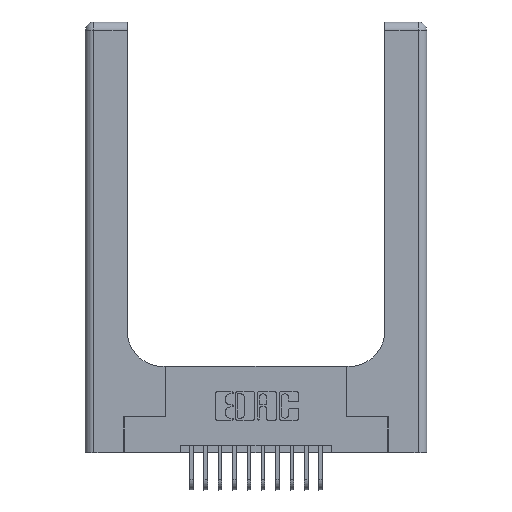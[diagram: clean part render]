
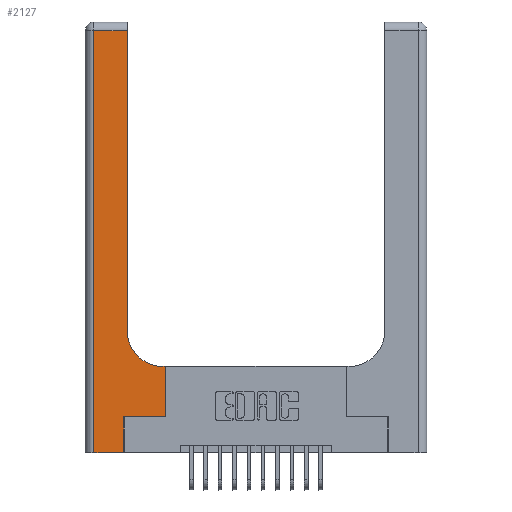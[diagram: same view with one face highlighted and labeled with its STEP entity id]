
A CAD part, top view. The second image highlights one B-rep face of the part: STEP entity #2127.
In plain terms, the highlighted planar face has unit normal (0, 0, 1).
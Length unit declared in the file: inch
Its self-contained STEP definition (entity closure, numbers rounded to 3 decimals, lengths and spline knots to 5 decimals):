
#463 = VERTEX_POINT ( 'NONE', #16548 ) ;
#672 = VERTEX_POINT ( 'NONE', #14677 ) ;
#1112 = VERTEX_POINT ( 'NONE', #16464 ) ;
#1236 = VECTOR ( 'NONE', #17780, 39.37008 ) ;
#1270 = CARTESIAN_POINT ( 'NONE',  ( 0.269, 0., 0.37 ) ) ;
#1528 = EDGE_CURVE ( 'NONE', #463, #9637, #14666, .T. ) ;
#1579 = VECTOR ( 'NONE', #14636, 39.37008 ) ;
#1701 = VECTOR ( 'NONE', #14413, 39.37008 ) ;
#1878 = VERTEX_POINT ( 'NONE', #7580 ) ;
#2127 = ADVANCED_FACE ( 'NONE', ( #17634 ), #6826, .F. ) ;
#2381 = LINE ( 'NONE', #10293, #9629 ) ;
#2548 = EDGE_CURVE ( 'NONE', #1112, #5466, #13866, .T. ) ;
#2613 = EDGE_LOOP ( 'NONE', ( #13103, #8641, #13406, #6641, #18690, #15716, #16175, #10915, #14862 ) ) ;
#3111 = VECTOR ( 'NONE', #7740, 39.37008 ) ;
#3195 = DIRECTION ( 'NONE',  ( -1., 0., 0. ) ) ;
#3203 = VECTOR ( 'NONE', #11678, 39.37008 ) ;
#3715 = VERTEX_POINT ( 'NONE', #17293 ) ;
#4484 = CARTESIAN_POINT ( 'NONE',  ( 0.5585, 0.25, 0.37 ) ) ;
#4715 = LINE ( 'NONE', #7609, #1236 ) ;
#4945 = CARTESIAN_POINT ( 'NONE',  ( 0.2915, 0.85, 0.37 ) ) ;
#5001 = EDGE_CURVE ( 'NONE', #3715, #1112, #16762, .T. ) ;
#5064 = LINE ( 'NONE', #16129, #1579 ) ;
#5176 = CARTESIAN_POINT ( 'NONE',  ( 0., 3., 0.37 ) ) ;
#5466 = VERTEX_POINT ( 'NONE', #4945 ) ;
#5770 = CARTESIAN_POINT ( 'NONE',  ( 0.2915, 0.6, 0.37 ) ) ;
#5920 = CARTESIAN_POINT ( 'NONE',  ( 0.269, 0., 0.37 ) ) ;
#6044 = DIRECTION ( 'NONE',  ( -1., 0., 0. ) ) ;
#6066 = LINE ( 'NONE', #11841, #12820 ) ;
#6090 = DIRECTION ( 'NONE',  ( 0., 0., -1. ) ) ;
#6641 = ORIENTED_EDGE ( 'NONE', *, *, #9458, .T. ) ;
#6823 = EDGE_CURVE ( 'NONE', #5466, #1878, #2381, .T. ) ;
#6826 = PLANE ( 'NONE',  #17528 ) ;
#6923 = DIRECTION ( 'NONE',  ( 0., 0., -1. ) ) ;
#7580 = CARTESIAN_POINT ( 'NONE',  ( 0.2915, 2.94, 0.37 ) ) ;
#7609 = CARTESIAN_POINT ( 'NONE',  ( 0.269, 0.25, 0.37 ) ) ;
#7680 = CARTESIAN_POINT ( 'NONE',  ( 0.06, 3., 0.37 ) ) ;
#7740 = DIRECTION ( 'NONE',  ( 0., -1., 0. ) ) ;
#8641 = ORIENTED_EDGE ( 'NONE', *, *, #18511, .T. ) ;
#8667 = LINE ( 'NONE', #5920, #15960 ) ;
#8853 = DIRECTION ( 'NONE',  ( 0., 1., 0. ) ) ;
#9458 = EDGE_CURVE ( 'NONE', #9637, #17975, #5064, .T. ) ;
#9629 = VECTOR ( 'NONE', #8853, 39.37008 ) ;
#9637 = VERTEX_POINT ( 'NONE', #17961 ) ;
#10058 = EDGE_CURVE ( 'NONE', #672, #3715, #14762, .T. ) ;
#10293 = CARTESIAN_POINT ( 'NONE',  ( 0.2915, 3., 0.37 ) ) ;
#10783 = CARTESIAN_POINT ( 'NONE',  ( 0.269, 0.25, 0.37 ) ) ;
#10915 = ORIENTED_EDGE ( 'NONE', *, *, #5001, .T. ) ;
#11678 = DIRECTION ( 'NONE',  ( 0., 1., 0. ) ) ;
#11841 = CARTESIAN_POINT ( 'NONE',  ( 0., 2.94, 0.37 ) ) ;
#12127 = EDGE_CURVE ( 'NONE', #12797, #672, #4715, .T. ) ;
#12797 = VERTEX_POINT ( 'NONE', #10783 ) ;
#12820 = VECTOR ( 'NONE', #3195, 39.37008 ) ;
#13103 = ORIENTED_EDGE ( 'NONE', *, *, #6823, .T. ) ;
#13406 = ORIENTED_EDGE ( 'NONE', *, *, #1528, .T. ) ;
#13866 = CIRCLE ( 'NONE', #17174, 0.25 ) ;
#14413 = DIRECTION ( 'NONE',  ( -1., 0., 0. ) ) ;
#14636 = DIRECTION ( 'NONE',  ( 1., 0., 0. ) ) ;
#14666 = LINE ( 'NONE', #7680, #3111 ) ;
#14677 = CARTESIAN_POINT ( 'NONE',  ( 0.5585, 0.25, 0.37 ) ) ;
#14762 = LINE ( 'NONE', #4484, #3203 ) ;
#14862 = ORIENTED_EDGE ( 'NONE', *, *, #2548, .T. ) ;
#15327 = EDGE_CURVE ( 'NONE', #17975, #12797, #8667, .T. ) ;
#15613 = CARTESIAN_POINT ( 'NONE',  ( 0.5415, 0.85, 0.37 ) ) ;
#15716 = ORIENTED_EDGE ( 'NONE', *, *, #12127, .T. ) ;
#15960 = VECTOR ( 'NONE', #17519, 39.37008 ) ;
#16129 = CARTESIAN_POINT ( 'NONE',  ( 0., 0., 0.37 ) ) ;
#16175 = ORIENTED_EDGE ( 'NONE', *, *, #10058, .T. ) ;
#16464 = CARTESIAN_POINT ( 'NONE',  ( 0.5415, 0.6, 0.37 ) ) ;
#16548 = CARTESIAN_POINT ( 'NONE',  ( 0.06, 2.94, 0.37 ) ) ;
#16762 = LINE ( 'NONE', #5770, #1701 ) ;
#17085 = DIRECTION ( 'NONE',  ( 1., 0., 0. ) ) ;
#17174 = AXIS2_PLACEMENT_3D ( 'NONE', #15613, #6923, #17085 ) ;
#17293 = CARTESIAN_POINT ( 'NONE',  ( 0.5585, 0.6, 0.37 ) ) ;
#17519 = DIRECTION ( 'NONE',  ( 0., 1., 0. ) ) ;
#17528 = AXIS2_PLACEMENT_3D ( 'NONE', #5176, #6090, #6044 ) ;
#17634 = FACE_OUTER_BOUND ( 'NONE', #2613, .T. ) ;
#17780 = DIRECTION ( 'NONE',  ( 1., 0., 0. ) ) ;
#17961 = CARTESIAN_POINT ( 'NONE',  ( 0.06, 0., 0.37 ) ) ;
#17975 = VERTEX_POINT ( 'NONE', #1270 ) ;
#18511 = EDGE_CURVE ( 'NONE', #1878, #463, #6066, .T. ) ;
#18690 = ORIENTED_EDGE ( 'NONE', *, *, #15327, .T. ) ;
